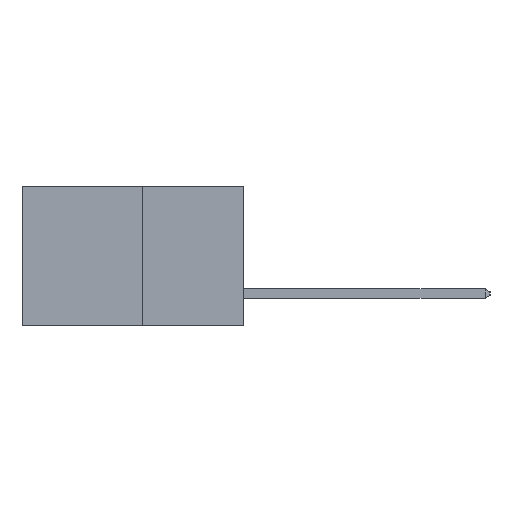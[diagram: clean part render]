
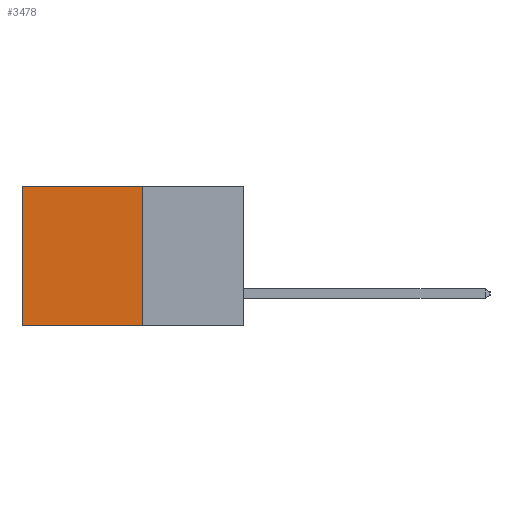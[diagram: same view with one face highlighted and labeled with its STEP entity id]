
A CAD part, left-side view. The second image highlights one B-rep face of the part: STEP entity #3478.
In plain terms, the highlighted planar face has unit normal (-1, 0, 0).
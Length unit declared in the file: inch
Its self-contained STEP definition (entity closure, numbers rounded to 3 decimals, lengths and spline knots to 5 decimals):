
#95 = VECTOR ( 'NONE', #6744, 39.37008 ) ;
#273 = CARTESIAN_POINT ( 'NONE',  ( 0.277, 0.59, -0.37 ) ) ;
#1025 = CARTESIAN_POINT ( 'NONE',  ( 0.277, 0.27, 0. ) ) ;
#1181 = DIRECTION ( 'NONE',  ( 0., 1., 0. ) ) ;
#1423 = VERTEX_POINT ( 'NONE', #273 ) ;
#1793 = VECTOR ( 'NONE', #2344, 39.37008 ) ;
#2321 = ORIENTED_EDGE ( 'NONE', *, *, #3319, .T. ) ;
#2344 = DIRECTION ( 'NONE',  ( 0., 1., 0. ) ) ;
#2421 = CARTESIAN_POINT ( 'NONE',  ( 0.277, 0.27, -0.37 ) ) ;
#2540 = FACE_OUTER_BOUND ( 'NONE', #5285, .T. ) ;
#2708 = VERTEX_POINT ( 'NONE', #7185 ) ;
#3047 = VERTEX_POINT ( 'NONE', #8089 ) ;
#3319 = EDGE_CURVE ( 'NONE', #4251, #2708, #4749, .T. ) ;
#3478 = ADVANCED_FACE ( 'NONE', ( #2540 ), #9573, .F. ) ;
#3964 = LINE ( 'NONE', #2421, #1793 ) ;
#4094 = VECTOR ( 'NONE', #6956, 39.37008 ) ;
#4251 = VERTEX_POINT ( 'NONE', #4905 ) ;
#4276 = AXIS2_PLACEMENT_3D ( 'NONE', #9664, #9559, #9548 ) ;
#4467 = ORIENTED_EDGE ( 'NONE', *, *, #4915, .F. ) ;
#4749 = LINE ( 'NONE', #1025, #8739 ) ;
#4905 = CARTESIAN_POINT ( 'NONE',  ( 0.277, 0.27, 0. ) ) ;
#4915 = EDGE_CURVE ( 'NONE', #3047, #1423, #3964, .T. ) ;
#5111 = LINE ( 'NONE', #6888, #95 ) ;
#5285 = EDGE_LOOP ( 'NONE', ( #10375, #4467, #10583, #2321 ) ) ;
#5964 = EDGE_CURVE ( 'NONE', #2708, #1423, #5111, .T. ) ;
#6245 = LINE ( 'NONE', #9494, #4094 ) ;
#6532 = EDGE_CURVE ( 'NONE', #4251, #3047, #6245, .T. ) ;
#6744 = DIRECTION ( 'NONE',  ( 0., 0., -1. ) ) ;
#6888 = CARTESIAN_POINT ( 'NONE',  ( 0.277, 0.59, -0.37 ) ) ;
#6956 = DIRECTION ( 'NONE',  ( 0., 0., -1. ) ) ;
#7185 = CARTESIAN_POINT ( 'NONE',  ( 0.277, 0.59, 0. ) ) ;
#8089 = CARTESIAN_POINT ( 'NONE',  ( 0.277, 0.27, -0.37 ) ) ;
#8739 = VECTOR ( 'NONE', #1181, 39.37008 ) ;
#9494 = CARTESIAN_POINT ( 'NONE',  ( 0.277, 0.27, -0.37 ) ) ;
#9548 = DIRECTION ( 'NONE',  ( 0., 0., -1. ) ) ;
#9559 = DIRECTION ( 'NONE',  ( 1., 0., 0. ) ) ;
#9573 = PLANE ( 'NONE',  #4276 ) ;
#9664 = CARTESIAN_POINT ( 'NONE',  ( 0.277, 0.27, -0.37 ) ) ;
#10375 = ORIENTED_EDGE ( 'NONE', *, *, #5964, .T. ) ;
#10583 = ORIENTED_EDGE ( 'NONE', *, *, #6532, .F. ) ;
